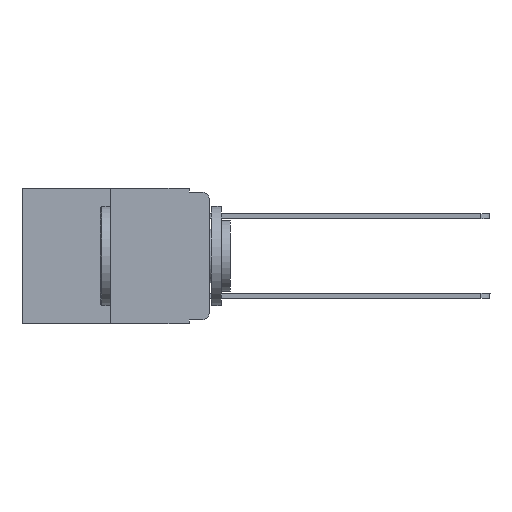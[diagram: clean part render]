
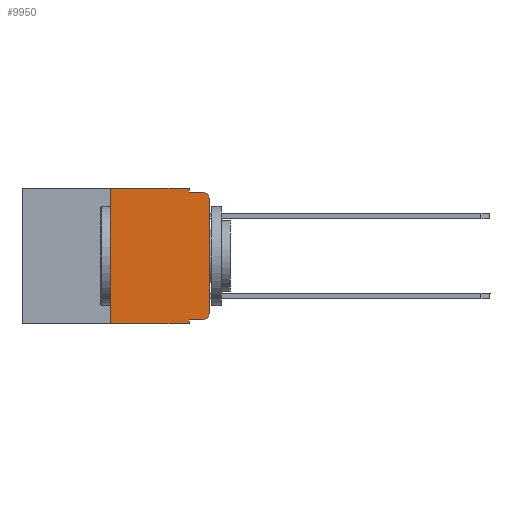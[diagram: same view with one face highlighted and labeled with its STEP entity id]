
A CAD part, left-side view. The second image highlights one B-rep face of the part: STEP entity #9950.
In plain terms, the highlighted planar face has unit normal (-1, 0, 0).
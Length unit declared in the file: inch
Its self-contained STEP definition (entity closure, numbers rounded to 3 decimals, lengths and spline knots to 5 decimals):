
#20 = ORIENTED_EDGE ( 'NONE', *, *, #6069, .T. ) ;
#57 = VERTEX_POINT ( 'NONE', #7470 ) ;
#83 = LINE ( 'NONE', #10601, #3010 ) ;
#130 = VERTEX_POINT ( 'NONE', #5710 ) ;
#274 = EDGE_CURVE ( 'NONE', #130, #5715, #4023, .T. ) ;
#791 = CARTESIAN_POINT ( 'NONE',  ( 0., 0., -0.313 ) ) ;
#849 = VERTEX_POINT ( 'NONE', #10142 ) ;
#1083 = DIRECTION ( 'NONE',  ( 0., -1., 0. ) ) ;
#1140 = DIRECTION ( 'NONE',  ( 0., -1., 0. ) ) ;
#1188 = VECTOR ( 'NONE', #11145, 39.37008 ) ;
#1300 = VECTOR ( 'NONE', #2225, 39.37008 ) ;
#1307 = CARTESIAN_POINT ( 'NONE',  ( 0., 0., 0. ) ) ;
#1604 = CARTESIAN_POINT ( 'NONE',  ( 0., 0.02, -0.313 ) ) ;
#1654 = EDGE_CURVE ( 'NONE', #5715, #10542, #4177, .T. ) ;
#1746 = VECTOR ( 'NONE', #10339, 39.37008 ) ;
#2202 = ORIENTED_EDGE ( 'NONE', *, *, #2951, .F. ) ;
#2225 = DIRECTION ( 'NONE',  ( 0., 0., -1. ) ) ;
#2672 = CARTESIAN_POINT ( 'NONE',  ( 0., 0.051, 0. ) ) ;
#2756 = CARTESIAN_POINT ( 'NONE',  ( 0., 0.25, 0. ) ) ;
#2874 = EDGE_CURVE ( 'NONE', #57, #9107, #10901, .T. ) ;
#2951 = EDGE_CURVE ( 'NONE', #849, #7533, #3155, .T. ) ;
#3010 = VECTOR ( 'NONE', #1083, 39.37008 ) ;
#3101 = AXIS2_PLACEMENT_3D ( 'NONE', #6794, #7806, #7746 ) ;
#3131 = VECTOR ( 'NONE', #11804, 39.37008 ) ;
#3155 = LINE ( 'NONE', #3410, #9917 ) ;
#3405 = CARTESIAN_POINT ( 'NONE',  ( 0., 0.051, 0. ) ) ;
#3410 = CARTESIAN_POINT ( 'NONE',  ( 0., 0.051, 0. ) ) ;
#3451 = CARTESIAN_POINT ( 'NONE',  ( 0., 0.051, -0.01 ) ) ;
#3563 = CARTESIAN_POINT ( 'NONE',  ( 0., 0.25, -0.343 ) ) ;
#3942 = ORIENTED_EDGE ( 'NONE', *, *, #1654, .F. ) ;
#4023 = LINE ( 'NONE', #7843, #8397 ) ;
#4177 = LINE ( 'NONE', #3405, #1300 ) ;
#4426 = DIRECTION ( 'NONE',  ( 0., 0., -1. ) ) ;
#4798 = EDGE_CURVE ( 'NONE', #9140, #130, #12259, .T. ) ;
#5110 = LINE ( 'NONE', #6107, #3131 ) ;
#5121 = DIRECTION ( 'NONE',  ( 0., 0., 1. ) ) ;
#5171 = AXIS2_PLACEMENT_3D ( 'NONE', #1604, #8366, #6479 ) ;
#5390 = CARTESIAN_POINT ( 'NONE',  ( 0., 0.02, -0.333 ) ) ;
#5710 = CARTESIAN_POINT ( 'NONE',  ( 0., 0.25, 0. ) ) ;
#5715 = VERTEX_POINT ( 'NONE', #2672 ) ;
#5727 = ORIENTED_EDGE ( 'NONE', *, *, #274, .F. ) ;
#6011 = VECTOR ( 'NONE', #5121, 39.37008 ) ;
#6069 = EDGE_CURVE ( 'NONE', #849, #9019, #5110, .T. ) ;
#6107 = CARTESIAN_POINT ( 'NONE',  ( 0., 0.051, -0.333 ) ) ;
#6219 = AXIS2_PLACEMENT_3D ( 'NONE', #9187, #7991, #4426 ) ;
#6479 = DIRECTION ( 'NONE',  ( 0., 0., -1. ) ) ;
#6794 = CARTESIAN_POINT ( 'NONE',  ( 0., 0.02, -0.03 ) ) ;
#6900 = CARTESIAN_POINT ( 'NONE',  ( 0., 0.02, -0.01 ) ) ;
#7022 = ORIENTED_EDGE ( 'NONE', *, *, #7514, .T. ) ;
#7073 = LINE ( 'NONE', #3451, #1188 ) ;
#7236 = CARTESIAN_POINT ( 'NONE',  ( 0., 0.051, -0.343 ) ) ;
#7470 = CARTESIAN_POINT ( 'NONE',  ( 0., 0., -0.03 ) ) ;
#7514 = EDGE_CURVE ( 'NONE', #9019, #9648, #10567, .T. ) ;
#7533 = VERTEX_POINT ( 'NONE', #7236 ) ;
#7746 = DIRECTION ( 'NONE',  ( 0., 0., -1. ) ) ;
#7806 = DIRECTION ( 'NONE',  ( -1., 0., 0. ) ) ;
#7843 = CARTESIAN_POINT ( 'NONE',  ( 0., 0.473, 0. ) ) ;
#7991 = DIRECTION ( 'NONE',  ( 1., 0., 0. ) ) ;
#8309 = EDGE_LOOP ( 'NONE', ( #9129, #8806, #9091, #3942, #5727, #11901, #12220, #2202, #20, #7022 ) ) ;
#8325 = EDGE_CURVE ( 'NONE', #10542, #9107, #7073, .T. ) ;
#8366 = DIRECTION ( 'NONE',  ( -1., 0., 0. ) ) ;
#8397 = VECTOR ( 'NONE', #1140, 39.37008 ) ;
#8806 = ORIENTED_EDGE ( 'NONE', *, *, #2874, .T. ) ;
#9019 = VERTEX_POINT ( 'NONE', #5390 ) ;
#9067 = DIRECTION ( 'NONE',  ( 0., 0., -1. ) ) ;
#9091 = ORIENTED_EDGE ( 'NONE', *, *, #8325, .F. ) ;
#9107 = VERTEX_POINT ( 'NONE', #6900 ) ;
#9129 = ORIENTED_EDGE ( 'NONE', *, *, #9495, .T. ) ;
#9140 = VERTEX_POINT ( 'NONE', #3563 ) ;
#9187 = CARTESIAN_POINT ( 'NONE',  ( 0., 0.473, 0. ) ) ;
#9286 = CARTESIAN_POINT ( 'NONE',  ( 0., 0.051, -0.01 ) ) ;
#9495 = EDGE_CURVE ( 'NONE', #9648, #57, #9893, .T. ) ;
#9648 = VERTEX_POINT ( 'NONE', #791 ) ;
#9893 = LINE ( 'NONE', #1307, #6011 ) ;
#9917 = VECTOR ( 'NONE', #9067, 39.37008 ) ;
#9950 = ADVANCED_FACE ( 'NONE', ( #11977 ), #10115, .F. ) ;
#10115 = PLANE ( 'NONE',  #6219 ) ;
#10142 = CARTESIAN_POINT ( 'NONE',  ( 0., 0.051, -0.333 ) ) ;
#10261 = EDGE_CURVE ( 'NONE', #9140, #7533, #83, .T. ) ;
#10339 = DIRECTION ( 'NONE',  ( 0., 0., 1. ) ) ;
#10542 = VERTEX_POINT ( 'NONE', #9286 ) ;
#10567 = CIRCLE ( 'NONE', #5171, 0.02 ) ;
#10601 = CARTESIAN_POINT ( 'NONE',  ( 0., 0.473, -0.343 ) ) ;
#10901 = CIRCLE ( 'NONE', #3101, 0.02 ) ;
#11145 = DIRECTION ( 'NONE',  ( 0., -1., 0. ) ) ;
#11804 = DIRECTION ( 'NONE',  ( 0., -1., 0. ) ) ;
#11901 = ORIENTED_EDGE ( 'NONE', *, *, #4798, .F. ) ;
#11977 = FACE_OUTER_BOUND ( 'NONE', #8309, .T. ) ;
#12220 = ORIENTED_EDGE ( 'NONE', *, *, #10261, .T. ) ;
#12259 = LINE ( 'NONE', #2756, #1746 ) ;
